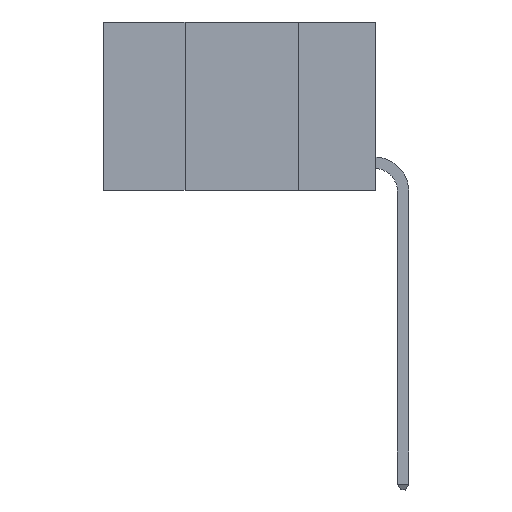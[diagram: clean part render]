
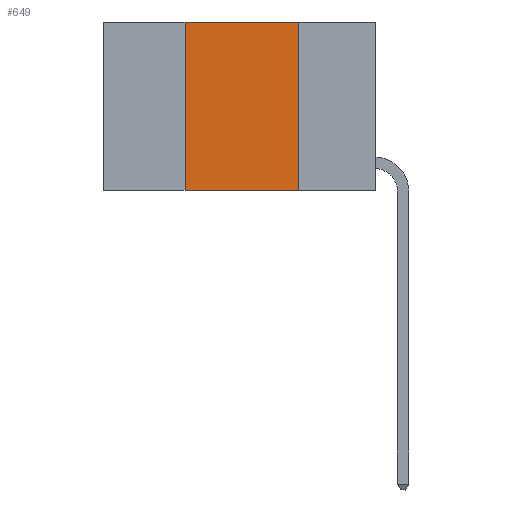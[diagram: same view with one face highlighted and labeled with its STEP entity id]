
A CAD part, left-side view. The second image highlights one B-rep face of the part: STEP entity #649.
In plain terms, the highlighted planar face has unit normal (-1, 0, 0).
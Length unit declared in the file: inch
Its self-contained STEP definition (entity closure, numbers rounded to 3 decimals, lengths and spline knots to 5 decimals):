
#344 = DIRECTION ( 'NONE',  ( 0., -1., 0. ) ) ;
#628 = CARTESIAN_POINT ( 'NONE',  ( 0., 0.6, 0. ) ) ;
#649 = ADVANCED_FACE ( 'NONE', ( #4769 ), #2547, .F. ) ;
#1338 = EDGE_CURVE ( 'NONE', #5979, #20517, #15398, .T. ) ;
#1891 = DIRECTION ( 'NONE',  ( 0., 0., 1. ) ) ;
#2547 = PLANE ( 'NONE',  #22263 ) ;
#4387 = VECTOR ( 'NONE', #344, 39.37008 ) ;
#4532 = VERTEX_POINT ( 'NONE', #14302 ) ;
#4676 = VECTOR ( 'NONE', #11384, 39.37008 ) ;
#4769 = FACE_OUTER_BOUND ( 'NONE', #15128, .T. ) ;
#4781 = DIRECTION ( 'NONE',  ( 0., 0., -1. ) ) ;
#5073 = LINE ( 'NONE', #16450, #26271 ) ;
#5979 = VERTEX_POINT ( 'NONE', #19063 ) ;
#8039 = CARTESIAN_POINT ( 'NONE',  ( 0., 0.17, 0. ) ) ;
#8596 = EDGE_CURVE ( 'NONE', #14407, #20517, #26289, .T. ) ;
#8925 = CARTESIAN_POINT ( 'NONE',  ( 0., 0.6, 0. ) ) ;
#9657 = EDGE_CURVE ( 'NONE', #4532, #14407, #16310, .T. ) ;
#11384 = DIRECTION ( 'NONE',  ( 0., -1., 0. ) ) ;
#14302 = CARTESIAN_POINT ( 'NONE',  ( 0., 0.42, 0. ) ) ;
#14407 = VERTEX_POINT ( 'NONE', #8039 ) ;
#15128 = EDGE_LOOP ( 'NONE', ( #20002, #26959, #24775, #20542 ) ) ;
#15398 = LINE ( 'NONE', #25291, #4387 ) ;
#15409 = VECTOR ( 'NONE', #20051, 39.37008 ) ;
#16310 = LINE ( 'NONE', #628, #4676 ) ;
#16450 = CARTESIAN_POINT ( 'NONE',  ( 0., 0.42, 0. ) ) ;
#17132 = DIRECTION ( 'NONE',  ( 1., 0., 0. ) ) ;
#18031 = CARTESIAN_POINT ( 'NONE',  ( 0., 0.17, 0. ) ) ;
#18178 = EDGE_CURVE ( 'NONE', #5979, #4532, #5073, .T. ) ;
#19063 = CARTESIAN_POINT ( 'NONE',  ( 0., 0.42, -0.37 ) ) ;
#20002 = ORIENTED_EDGE ( 'NONE', *, *, #8596, .F. ) ;
#20051 = DIRECTION ( 'NONE',  ( 0., 0., -1. ) ) ;
#20517 = VERTEX_POINT ( 'NONE', #26082 ) ;
#20542 = ORIENTED_EDGE ( 'NONE', *, *, #1338, .T. ) ;
#22263 = AXIS2_PLACEMENT_3D ( 'NONE', #8925, #17132, #4781 ) ;
#24775 = ORIENTED_EDGE ( 'NONE', *, *, #18178, .F. ) ;
#25291 = CARTESIAN_POINT ( 'NONE',  ( 0., 0.6, -0.37 ) ) ;
#26082 = CARTESIAN_POINT ( 'NONE',  ( 0., 0.17, -0.37 ) ) ;
#26271 = VECTOR ( 'NONE', #1891, 39.37008 ) ;
#26289 = LINE ( 'NONE', #18031, #15409 ) ;
#26959 = ORIENTED_EDGE ( 'NONE', *, *, #9657, .F. ) ;
